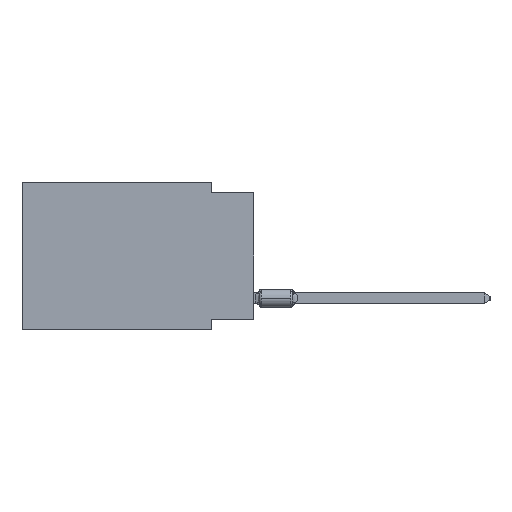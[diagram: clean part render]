
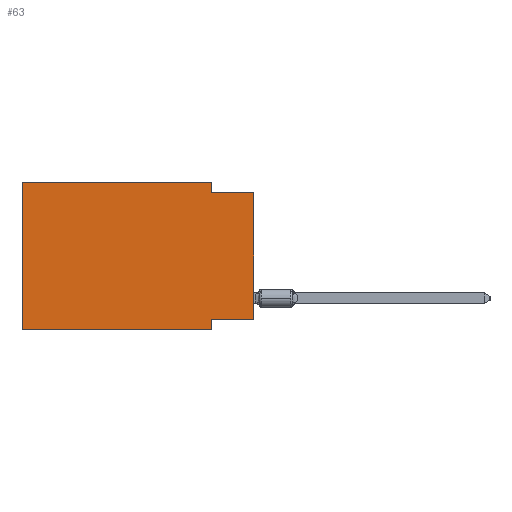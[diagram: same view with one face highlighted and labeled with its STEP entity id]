
A CAD part, left-side view. The second image highlights one B-rep face of the part: STEP entity #63.
In plain terms, the highlighted planar face has unit normal (-1, 0, 0).
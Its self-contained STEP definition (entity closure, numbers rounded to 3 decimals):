
#63 = ADVANCED_FACE ( 'NONE', ( #21512 ), #12781, .F. ) ;
#165 = LINE ( 'NONE', #8700, #30870 ) ;
#569 = VERTEX_POINT ( 'NONE', #27355 ) ;
#1000 = DIRECTION ( 'NONE',  ( 0., -1., 0. ) ) ;
#2495 = VECTOR ( 'NONE', #27965, 1000. ) ;
#2830 = CARTESIAN_POINT ( 'NONE',  ( 0., 0., -8.255 ) ) ;
#3226 = VECTOR ( 'NONE', #21069, 1000. ) ;
#3425 = EDGE_CURVE ( 'NONE', #569, #36011, #23511, .T. ) ;
#5232 = CARTESIAN_POINT ( 'NONE',  ( 0., 2.54, -0.635 ) ) ;
#5717 = CARTESIAN_POINT ( 'NONE',  ( 0., 2.54, 0. ) ) ;
#6300 = EDGE_CURVE ( 'NONE', #35906, #36011, #16196, .T. ) ;
#7276 = DIRECTION ( 'NONE',  ( 1., 0., 0. ) ) ;
#7564 = VECTOR ( 'NONE', #26738, 1000. ) ;
#8136 = EDGE_CURVE ( 'NONE', #8263, #35906, #12159, .T. ) ;
#8263 = VERTEX_POINT ( 'NONE', #2830 ) ;
#8264 = CARTESIAN_POINT ( 'NONE',  ( 0., 13.97, 0. ) ) ;
#8700 = CARTESIAN_POINT ( 'NONE',  ( 0., 0., -0.635 ) ) ;
#9531 = CARTESIAN_POINT ( 'NONE',  ( 0., 13.97, 0. ) ) ;
#10890 = AXIS2_PLACEMENT_3D ( 'NONE', #18846, #7276, #12973 ) ;
#10986 = EDGE_LOOP ( 'NONE', ( #11089, #34765, #31536, #16153, #30855, #16576, #35985, #12925 ) ) ;
#11089 = ORIENTED_EDGE ( 'NONE', *, *, #15732, .T. ) ;
#11190 = VERTEX_POINT ( 'NONE', #5232 ) ;
#12159 = LINE ( 'NONE', #26775, #3226 ) ;
#12781 = PLANE ( 'NONE',  #10890 ) ;
#12794 = VERTEX_POINT ( 'NONE', #26868 ) ;
#12925 = ORIENTED_EDGE ( 'NONE', *, *, #8136, .F. ) ;
#12973 = DIRECTION ( 'NONE',  ( 0., 0., -1. ) ) ;
#14589 = CARTESIAN_POINT ( 'NONE',  ( 0., 13.97, -8.89 ) ) ;
#15246 = VECTOR ( 'NONE', #26934, 1000. ) ;
#15358 = CARTESIAN_POINT ( 'NONE',  ( 0., 2.54, 0. ) ) ;
#15732 = EDGE_CURVE ( 'NONE', #8263, #12794, #16348, .T. ) ;
#16153 = ORIENTED_EDGE ( 'NONE', *, *, #23550, .F. ) ;
#16196 = LINE ( 'NONE', #27775, #2495 ) ;
#16348 = LINE ( 'NONE', #30774, #21345 ) ;
#16570 = DIRECTION ( 'NONE',  ( 0., 0., 1. ) ) ;
#16576 = ORIENTED_EDGE ( 'NONE', *, *, #3425, .T. ) ;
#17606 = DIRECTION ( 'NONE',  ( 0., -1., 0. ) ) ;
#18740 = LINE ( 'NONE', #15358, #15246 ) ;
#18846 = CARTESIAN_POINT ( 'NONE',  ( 0., 13.97, 0. ) ) ;
#19135 = CARTESIAN_POINT ( 'NONE',  ( 0., 2.54, -8.255 ) ) ;
#21069 = DIRECTION ( 'NONE',  ( 0., 1., 0. ) ) ;
#21345 = VECTOR ( 'NONE', #28299, 1000. ) ;
#21512 = FACE_OUTER_BOUND ( 'NONE', #10986, .T. ) ;
#21839 = VERTEX_POINT ( 'NONE', #8264 ) ;
#22194 = EDGE_CURVE ( 'NONE', #569, #21839, #33652, .T. ) ;
#23511 = LINE ( 'NONE', #14589, #7564 ) ;
#23550 = EDGE_CURVE ( 'NONE', #21839, #34402, #35542, .T. ) ;
#24970 = VECTOR ( 'NONE', #1000, 1000. ) ;
#26314 = VECTOR ( 'NONE', #16570, 1000. ) ;
#26738 = DIRECTION ( 'NONE',  ( 0., -1., 0. ) ) ;
#26775 = CARTESIAN_POINT ( 'NONE',  ( 0., 0., -8.255 ) ) ;
#26868 = CARTESIAN_POINT ( 'NONE',  ( 0., 0., -0.635 ) ) ;
#26934 = DIRECTION ( 'NONE',  ( 0., 0., -1. ) ) ;
#27355 = CARTESIAN_POINT ( 'NONE',  ( 0., 13.97, -8.89 ) ) ;
#27775 = CARTESIAN_POINT ( 'NONE',  ( 0., 2.54, -8.89 ) ) ;
#27965 = DIRECTION ( 'NONE',  ( 0., 0., -1. ) ) ;
#28299 = DIRECTION ( 'NONE',  ( 0., 0., 1. ) ) ;
#28621 = CARTESIAN_POINT ( 'NONE',  ( 0., 2.54, -8.89 ) ) ;
#28817 = EDGE_CURVE ( 'NONE', #34402, #11190, #18740, .T. ) ;
#30774 = CARTESIAN_POINT ( 'NONE',  ( 0., 0., 0. ) ) ;
#30855 = ORIENTED_EDGE ( 'NONE', *, *, #22194, .F. ) ;
#30870 = VECTOR ( 'NONE', #17606, 1000. ) ;
#31536 = ORIENTED_EDGE ( 'NONE', *, *, #28817, .F. ) ;
#33652 = LINE ( 'NONE', #36303, #26314 ) ;
#34402 = VERTEX_POINT ( 'NONE', #5717 ) ;
#34765 = ORIENTED_EDGE ( 'NONE', *, *, #36054, .F. ) ;
#35542 = LINE ( 'NONE', #9531, #24970 ) ;
#35906 = VERTEX_POINT ( 'NONE', #19135 ) ;
#35985 = ORIENTED_EDGE ( 'NONE', *, *, #6300, .F. ) ;
#36011 = VERTEX_POINT ( 'NONE', #28621 ) ;
#36054 = EDGE_CURVE ( 'NONE', #11190, #12794, #165, .T. ) ;
#36303 = CARTESIAN_POINT ( 'NONE',  ( 0., 13.97, 0. ) ) ;
